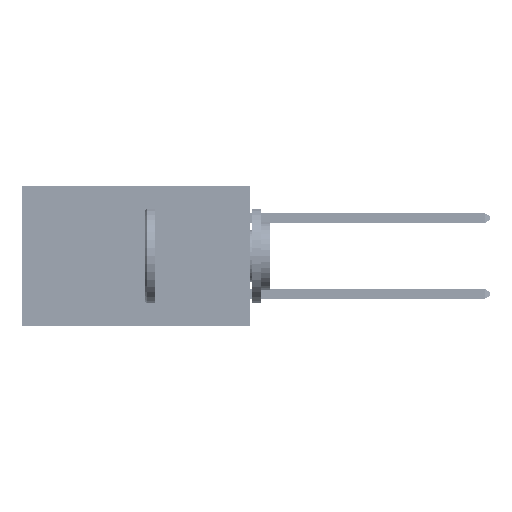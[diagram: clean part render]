
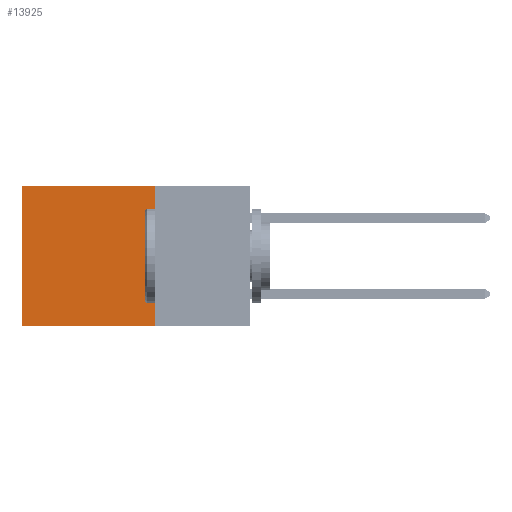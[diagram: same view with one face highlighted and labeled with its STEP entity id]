
A CAD part, left-side view. The second image highlights one B-rep face of the part: STEP entity #13925.
In plain terms, the highlighted planar face has unit normal (-1, 0, 0).
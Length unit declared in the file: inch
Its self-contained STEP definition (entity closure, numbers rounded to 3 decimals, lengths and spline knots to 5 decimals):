
#911 = LINE ( 'NONE', #8674, #41907 ) ;
#2066 = LINE ( 'NONE', #8212, #17740 ) ;
#4845 = ORIENTED_EDGE ( 'NONE', *, *, #9386, .F. ) ;
#5438 = PLANE ( 'NONE',  #27406 ) ;
#5727 = EDGE_LOOP ( 'NONE', ( #34976, #4845, #20019, #9609 ) ) ;
#7027 = VERTEX_POINT ( 'NONE', #9394 ) ;
#8212 = CARTESIAN_POINT ( 'NONE',  ( 0.2875, 0.25, 0. ) ) ;
#8674 = CARTESIAN_POINT ( 'NONE',  ( 0.2875, 0.25, -0.37 ) ) ;
#8782 = CARTESIAN_POINT ( 'NONE',  ( 0.2875, 0.25, 0. ) ) ;
#9386 = EDGE_CURVE ( 'NONE', #7027, #34113, #911, .T. ) ;
#9394 = CARTESIAN_POINT ( 'NONE',  ( 0.2875, 0.25, -0.37 ) ) ;
#9609 = ORIENTED_EDGE ( 'NONE', *, *, #41283, .T. ) ;
#10709 = LINE ( 'NONE', #38796, #26398 ) ;
#13191 = DIRECTION ( 'NONE',  ( 0., 0., -1. ) ) ;
#13925 = ADVANCED_FACE ( 'NONE', ( #40021 ), #5438, .F. ) ;
#16138 = DIRECTION ( 'NONE',  ( 0., 1., 0. ) ) ;
#16352 = DIRECTION ( 'NONE',  ( 1., 0., 0. ) ) ;
#17740 = VECTOR ( 'NONE', #16138, 39.37008 ) ;
#20019 = ORIENTED_EDGE ( 'NONE', *, *, #23822, .F. ) ;
#20458 = CARTESIAN_POINT ( 'NONE',  ( 0.2875, 0.25, 0. ) ) ;
#21815 = CARTESIAN_POINT ( 'NONE',  ( 0.2875, 0.6, -0.37 ) ) ;
#23822 = EDGE_CURVE ( 'NONE', #25093, #7027, #39500, .T. ) ;
#24441 = CARTESIAN_POINT ( 'NONE',  ( 0.2875, 0.25, 0. ) ) ;
#25093 = VERTEX_POINT ( 'NONE', #24441 ) ;
#26398 = VECTOR ( 'NONE', #42337, 39.37008 ) ;
#27406 = AXIS2_PLACEMENT_3D ( 'NONE', #8782, #16352, #13191 ) ;
#28092 = DIRECTION ( 'NONE',  ( 0., 0., -1. ) ) ;
#31615 = CARTESIAN_POINT ( 'NONE',  ( 0.2875, 0.6, 0. ) ) ;
#33505 = VECTOR ( 'NONE', #28092, 39.37008 ) ;
#34113 = VERTEX_POINT ( 'NONE', #21815 ) ;
#34976 = ORIENTED_EDGE ( 'NONE', *, *, #36362, .T. ) ;
#35289 = DIRECTION ( 'NONE',  ( 0., 1., 0. ) ) ;
#36362 = EDGE_CURVE ( 'NONE', #43643, #34113, #10709, .T. ) ;
#38796 = CARTESIAN_POINT ( 'NONE',  ( 0.2875, 0.6, 0. ) ) ;
#39500 = LINE ( 'NONE', #20458, #33505 ) ;
#40021 = FACE_OUTER_BOUND ( 'NONE', #5727, .T. ) ;
#41283 = EDGE_CURVE ( 'NONE', #25093, #43643, #2066, .T. ) ;
#41907 = VECTOR ( 'NONE', #35289, 39.37008 ) ;
#42337 = DIRECTION ( 'NONE',  ( 0., 0., -1. ) ) ;
#43643 = VERTEX_POINT ( 'NONE', #31615 ) ;
